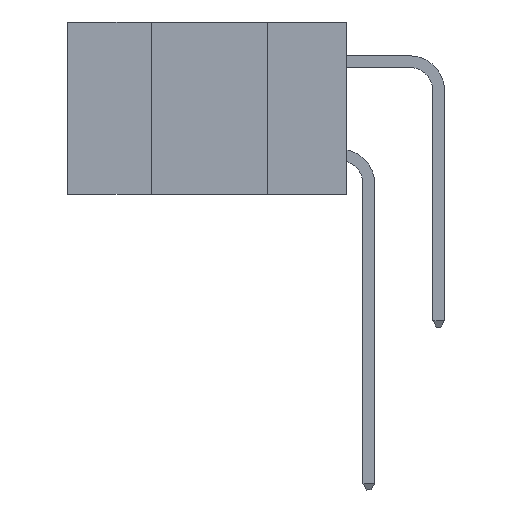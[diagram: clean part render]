
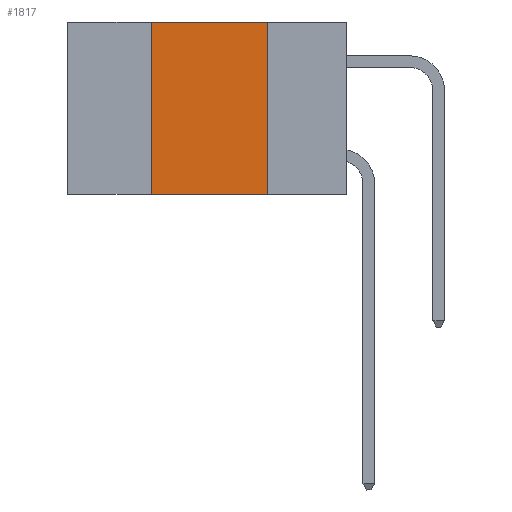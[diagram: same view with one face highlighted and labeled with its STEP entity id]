
A CAD part, left-side view. The second image highlights one B-rep face of the part: STEP entity #1817.
In plain terms, the highlighted planar face has unit normal (-1, 0, 0).
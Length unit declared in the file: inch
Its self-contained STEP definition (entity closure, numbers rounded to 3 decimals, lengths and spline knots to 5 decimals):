
#5 = EDGE_LOOP ( 'NONE', ( #12196, #12289, #12364, #12375 ) ) ;
#904 = EDGE_CURVE ( 'NONE', #1107, #5883, #974, .T. ) ;
#974 = LINE ( 'NONE', #3485, #3157 ) ;
#1107 = VERTEX_POINT ( 'NONE', #5409 ) ;
#1817 = ADVANCED_FACE ( 'NONE', ( #7499 ), #3234, .F. ) ;
#1891 = EDGE_CURVE ( 'NONE', #1107, #6151, #9117, .T. ) ;
#1928 = CARTESIAN_POINT ( 'NONE',  ( 0., 0.6, 0. ) ) ;
#1950 = CARTESIAN_POINT ( 'NONE',  ( 0., 0.6, -0.37 ) ) ;
#3091 = DIRECTION ( 'NONE',  ( 1., 0., 0. ) ) ;
#3157 = VECTOR ( 'NONE', #5141, 39.37008 ) ;
#3234 = PLANE ( 'NONE',  #10450 ) ;
#3253 = DIRECTION ( 'NONE',  ( 0., -1., 0. ) ) ;
#3349 = CARTESIAN_POINT ( 'NONE',  ( 0., 0.17, 0. ) ) ;
#3357 = DIRECTION ( 'NONE',  ( 0., 0., -1. ) ) ;
#3485 = CARTESIAN_POINT ( 'NONE',  ( 0., 0.42, 0. ) ) ;
#4971 = CARTESIAN_POINT ( 'NONE',  ( 0., 0.42, 0. ) ) ;
#5141 = DIRECTION ( 'NONE',  ( 0., 0., 1. ) ) ;
#5409 = CARTESIAN_POINT ( 'NONE',  ( 0., 0.42, -0.37 ) ) ;
#5883 = VERTEX_POINT ( 'NONE', #4971 ) ;
#6151 = VERTEX_POINT ( 'NONE', #10048 ) ;
#6240 = EDGE_CURVE ( 'NONE', #5883, #11063, #8637, .T. ) ;
#6626 = VECTOR ( 'NONE', #3253, 39.37008 ) ;
#7404 = DIRECTION ( 'NONE',  ( 0., -1., 0. ) ) ;
#7499 = FACE_OUTER_BOUND ( 'NONE', #5, .T. ) ;
#8637 = LINE ( 'NONE', #10169, #11997 ) ;
#9117 = LINE ( 'NONE', #1950, #6626 ) ;
#10048 = CARTESIAN_POINT ( 'NONE',  ( 0., 0.17, -0.37 ) ) ;
#10169 = CARTESIAN_POINT ( 'NONE',  ( 0., 0.6, 0. ) ) ;
#10210 = EDGE_CURVE ( 'NONE', #11063, #6151, #10394, .T. ) ;
#10394 = LINE ( 'NONE', #3349, #12464 ) ;
#10450 = AXIS2_PLACEMENT_3D ( 'NONE', #1928, #3091, #3357 ) ;
#10858 = DIRECTION ( 'NONE',  ( 0., 0., -1. ) ) ;
#10977 = CARTESIAN_POINT ( 'NONE',  ( 0., 0.17, 0. ) ) ;
#11063 = VERTEX_POINT ( 'NONE', #10977 ) ;
#11997 = VECTOR ( 'NONE', #7404, 39.37008 ) ;
#12196 = ORIENTED_EDGE ( 'NONE', *, *, #10210, .F. ) ;
#12289 = ORIENTED_EDGE ( 'NONE', *, *, #6240, .F. ) ;
#12364 = ORIENTED_EDGE ( 'NONE', *, *, #904, .F. ) ;
#12375 = ORIENTED_EDGE ( 'NONE', *, *, #1891, .T. ) ;
#12464 = VECTOR ( 'NONE', #10858, 39.37008 ) ;
